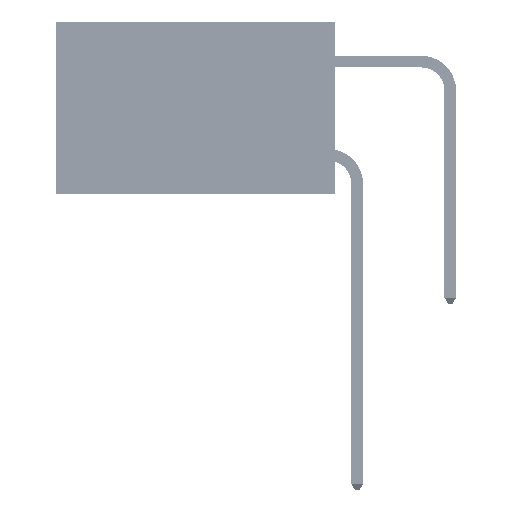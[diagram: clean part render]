
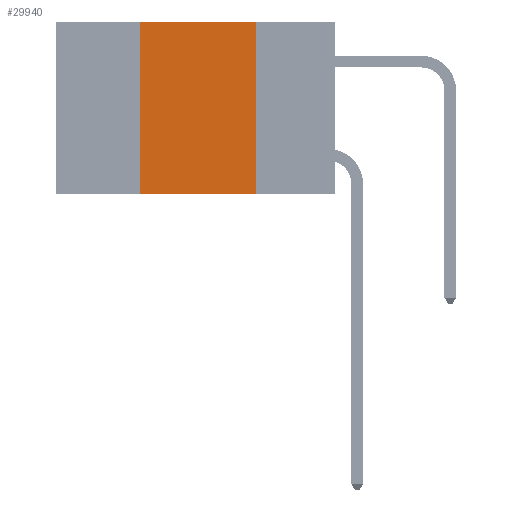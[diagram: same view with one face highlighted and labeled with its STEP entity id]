
A CAD part, left-side view. The second image highlights one B-rep face of the part: STEP entity #29940.
In plain terms, the highlighted planar face has unit normal (-1, 0, 0).
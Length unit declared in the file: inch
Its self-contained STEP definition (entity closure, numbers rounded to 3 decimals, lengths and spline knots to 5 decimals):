
#1 = DIRECTION ( 'NONE',  ( 0., 0., 1. ) ) ;
#1663 = EDGE_LOOP ( 'NONE', ( #48272, #24717, #21004, #39002 ) ) ;
#2679 = DIRECTION ( 'NONE',  ( 0., 0., -1. ) ) ;
#6000 = LINE ( 'NONE', #25674, #42230 ) ;
#6034 = CARTESIAN_POINT ( 'NONE',  ( 0., 0.6, 0. ) ) ;
#6521 = DIRECTION ( 'NONE',  ( 0., -1., 0. ) ) ;
#9619 = DIRECTION ( 'NONE',  ( 1., 0., 0. ) ) ;
#12515 = LINE ( 'NONE', #30029, #37623 ) ;
#13379 = DIRECTION ( 'NONE',  ( 0., 0., -1. ) ) ;
#13990 = VERTEX_POINT ( 'NONE', #17345 ) ;
#15402 = VERTEX_POINT ( 'NONE', #41945 ) ;
#17345 = CARTESIAN_POINT ( 'NONE',  ( 0., 0.42, 0. ) ) ;
#19901 = VECTOR ( 'NONE', #40850, 39.37008 ) ;
#20130 = EDGE_CURVE ( 'NONE', #13990, #27653, #26045, .T. ) ;
#20332 = EDGE_CURVE ( 'NONE', #26346, #15402, #12515, .T. ) ;
#21004 = ORIENTED_EDGE ( 'NONE', *, *, #25755, .F. ) ;
#21343 = CARTESIAN_POINT ( 'NONE',  ( 0., 0.42, -0.37 ) ) ;
#24717 = ORIENTED_EDGE ( 'NONE', *, *, #20130, .F. ) ;
#25198 = CARTESIAN_POINT ( 'NONE',  ( 0., 0.17, 0. ) ) ;
#25674 = CARTESIAN_POINT ( 'NONE',  ( 0., 0.17, 0. ) ) ;
#25755 = EDGE_CURVE ( 'NONE', #26346, #13990, #26154, .T. ) ;
#26045 = LINE ( 'NONE', #6034, #19901 ) ;
#26154 = LINE ( 'NONE', #43442, #28011 ) ;
#26346 = VERTEX_POINT ( 'NONE', #21343 ) ;
#27653 = VERTEX_POINT ( 'NONE', #25198 ) ;
#28011 = VECTOR ( 'NONE', #1, 39.37008 ) ;
#29007 = PLANE ( 'NONE',  #37135 ) ;
#29940 = ADVANCED_FACE ( 'NONE', ( #45574 ), #29007, .F. ) ;
#30029 = CARTESIAN_POINT ( 'NONE',  ( 0., 0.6, -0.37 ) ) ;
#31892 = EDGE_CURVE ( 'NONE', #27653, #15402, #6000, .T. ) ;
#37135 = AXIS2_PLACEMENT_3D ( 'NONE', #37208, #9619, #13379 ) ;
#37208 = CARTESIAN_POINT ( 'NONE',  ( 0., 0.6, 0. ) ) ;
#37623 = VECTOR ( 'NONE', #6521, 39.37008 ) ;
#39002 = ORIENTED_EDGE ( 'NONE', *, *, #20332, .T. ) ;
#40850 = DIRECTION ( 'NONE',  ( 0., -1., 0. ) ) ;
#41945 = CARTESIAN_POINT ( 'NONE',  ( 0., 0.17, -0.37 ) ) ;
#42230 = VECTOR ( 'NONE', #2679, 39.37008 ) ;
#43442 = CARTESIAN_POINT ( 'NONE',  ( 0., 0.42, 0. ) ) ;
#45574 = FACE_OUTER_BOUND ( 'NONE', #1663, .T. ) ;
#48272 = ORIENTED_EDGE ( 'NONE', *, *, #31892, .F. ) ;
